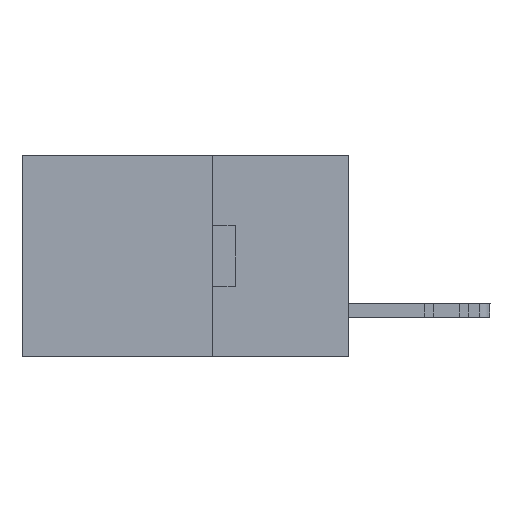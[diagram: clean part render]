
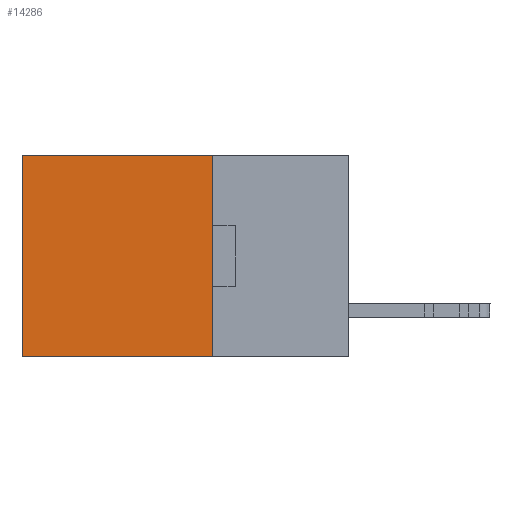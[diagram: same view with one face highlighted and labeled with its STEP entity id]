
A CAD part, left-side view. The second image highlights one B-rep face of the part: STEP entity #14286.
In plain terms, the highlighted planar face has unit normal (-1, 0, 0).
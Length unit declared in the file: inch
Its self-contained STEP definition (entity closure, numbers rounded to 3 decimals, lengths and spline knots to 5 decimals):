
#367 = ORIENTED_EDGE ( 'NONE', *, *, #25238, .F. ) ;
#1785 = CARTESIAN_POINT ( 'NONE',  ( 0.2615, 0.25, -0.37 ) ) ;
#1855 = VECTOR ( 'NONE', #9164, 39.37008 ) ;
#3864 = DIRECTION ( 'NONE',  ( 0., 0., -1. ) ) ;
#3964 = ORIENTED_EDGE ( 'NONE', *, *, #9019, .T. ) ;
#4736 = EDGE_CURVE ( 'NONE', #17013, #11158, #4876, .T. ) ;
#4876 = LINE ( 'NONE', #14374, #10307 ) ;
#5569 = CARTESIAN_POINT ( 'NONE',  ( 0.2615, 0.25, -0.37 ) ) ;
#7071 = DIRECTION ( 'NONE',  ( 0., 0., -1. ) ) ;
#7809 = VERTEX_POINT ( 'NONE', #8147 ) ;
#7947 = PLANE ( 'NONE',  #22252 ) ;
#8147 = CARTESIAN_POINT ( 'NONE',  ( 0.2615, 0.6, -0.37 ) ) ;
#9019 = EDGE_CURVE ( 'NONE', #11158, #7809, #18897, .T. ) ;
#9164 = DIRECTION ( 'NONE',  ( 0., 0., -1. ) ) ;
#10307 = VECTOR ( 'NONE', #14076, 39.37008 ) ;
#11158 = VERTEX_POINT ( 'NONE', #21827 ) ;
#11316 = EDGE_CURVE ( 'NONE', #24284, #7809, #25607, .T. ) ;
#12191 = CARTESIAN_POINT ( 'NONE',  ( 0.2615, 0.25, -0.37 ) ) ;
#14076 = DIRECTION ( 'NONE',  ( 0., 1., 0. ) ) ;
#14282 = VECTOR ( 'NONE', #18264, 39.37008 ) ;
#14286 = ADVANCED_FACE ( 'NONE', ( #19824 ), #7947, .F. ) ;
#14374 = CARTESIAN_POINT ( 'NONE',  ( 0.2615, 0.25, 0. ) ) ;
#14609 = VECTOR ( 'NONE', #7071, 39.37008 ) ;
#16168 = DIRECTION ( 'NONE',  ( 1., 0., 0. ) ) ;
#17013 = VERTEX_POINT ( 'NONE', #22216 ) ;
#18254 = ORIENTED_EDGE ( 'NONE', *, *, #4736, .T. ) ;
#18264 = DIRECTION ( 'NONE',  ( 0., 1., 0. ) ) ;
#18897 = LINE ( 'NONE', #19371, #1855 ) ;
#19371 = CARTESIAN_POINT ( 'NONE',  ( 0.2615, 0.6, -0.37 ) ) ;
#19824 = FACE_OUTER_BOUND ( 'NONE', #20317, .T. ) ;
#20317 = EDGE_LOOP ( 'NONE', ( #3964, #20850, #367, #18254 ) ) ;
#20850 = ORIENTED_EDGE ( 'NONE', *, *, #11316, .F. ) ;
#21366 = CARTESIAN_POINT ( 'NONE',  ( 0.2615, 0.25, -0.37 ) ) ;
#21827 = CARTESIAN_POINT ( 'NONE',  ( 0.2615, 0.6, 0. ) ) ;
#22216 = CARTESIAN_POINT ( 'NONE',  ( 0.2615, 0.25, 0. ) ) ;
#22252 = AXIS2_PLACEMENT_3D ( 'NONE', #1785, #16168, #3864 ) ;
#24284 = VERTEX_POINT ( 'NONE', #5569 ) ;
#24709 = LINE ( 'NONE', #21366, #14609 ) ;
#25238 = EDGE_CURVE ( 'NONE', #17013, #24284, #24709, .T. ) ;
#25607 = LINE ( 'NONE', #12191, #14282 ) ;
